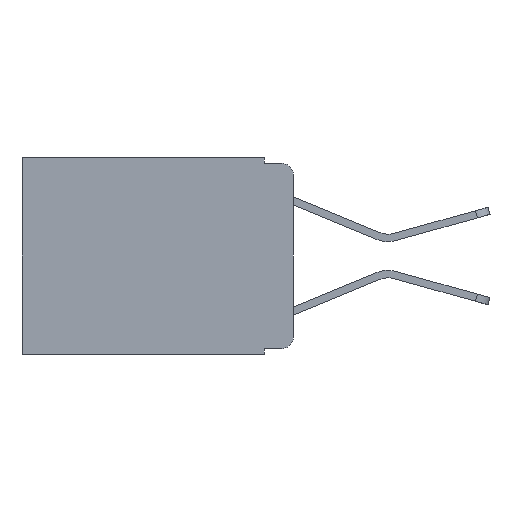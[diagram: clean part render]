
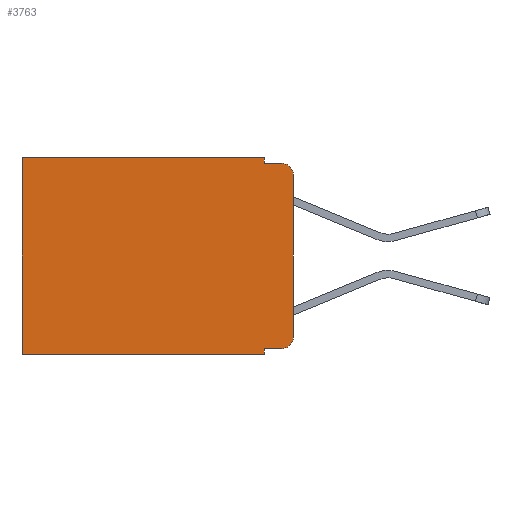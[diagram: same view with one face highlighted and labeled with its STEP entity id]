
A CAD part, left-side view. The second image highlights one B-rep face of the part: STEP entity #3763.
In plain terms, the highlighted planar face has unit normal (-1, 0, 0).
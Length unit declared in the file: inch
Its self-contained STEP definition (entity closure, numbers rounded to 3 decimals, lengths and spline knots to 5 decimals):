
#31 = ORIENTED_EDGE ( 'NONE', *, *, #11046, .F. ) ;
#92 = ORIENTED_EDGE ( 'NONE', *, *, #14139, .T. ) ;
#137 = CARTESIAN_POINT ( 'NONE',  ( 0.298, 0.051, -0.01 ) ) ;
#171 = ORIENTED_EDGE ( 'NONE', *, *, #2038, .T. ) ;
#335 = ORIENTED_EDGE ( 'NONE', *, *, #9919, .F. ) ;
#476 = VERTEX_POINT ( 'NONE', #11077 ) ;
#983 = LINE ( 'NONE', #5028, #12335 ) ;
#1116 = VECTOR ( 'NONE', #5757, 39.37008 ) ;
#1168 = EDGE_CURVE ( 'NONE', #7284, #14015, #10389, .T. ) ;
#1382 = DIRECTION ( 'NONE',  ( 0., 1., 0. ) ) ;
#1577 = DIRECTION ( 'NONE',  ( 0., 0., -1. ) ) ;
#1626 = VERTEX_POINT ( 'NONE', #10877 ) ;
#1864 = DIRECTION ( 'NONE',  ( 0., 1., 0. ) ) ;
#2035 = CARTESIAN_POINT ( 'NONE',  ( 0.298, 0.051, -0.333 ) ) ;
#2038 = EDGE_CURVE ( 'NONE', #14015, #6828, #9167, .T. ) ;
#2637 = CARTESIAN_POINT ( 'NONE',  ( 0.298, 0.473, 0. ) ) ;
#2832 = LINE ( 'NONE', #9396, #5446 ) ;
#3316 = CARTESIAN_POINT ( 'NONE',  ( 0.298, 0.051, -0.333 ) ) ;
#3537 = CARTESIAN_POINT ( 'NONE',  ( 0.298, 0.051, 0. ) ) ;
#3763 = ADVANCED_FACE ( 'NONE', ( #7193 ), #12557, .F. ) ;
#3995 = DIRECTION ( 'NONE',  ( 0., 0., -1. ) ) ;
#4475 = CARTESIAN_POINT ( 'NONE',  ( 0.298, 0., -0.313 ) ) ;
#4646 = ORIENTED_EDGE ( 'NONE', *, *, #6934, .T. ) ;
#4692 = CARTESIAN_POINT ( 'NONE',  ( 0.298, 0.02, -0.03 ) ) ;
#4764 = CARTESIAN_POINT ( 'NONE',  ( 0.298, 0.02, -0.333 ) ) ;
#4930 = VERTEX_POINT ( 'NONE', #6167 ) ;
#5028 = CARTESIAN_POINT ( 'NONE',  ( 0.298, 0., 0. ) ) ;
#5044 = CARTESIAN_POINT ( 'NONE',  ( 0.298, 0., -0.03 ) ) ;
#5356 = CARTESIAN_POINT ( 'NONE',  ( 0.298, 0., -0.343 ) ) ;
#5358 = DIRECTION ( 'NONE',  ( 0., -1., 0. ) ) ;
#5446 = VECTOR ( 'NONE', #1382, 39.37008 ) ;
#5665 = ORIENTED_EDGE ( 'NONE', *, *, #10648, .F. ) ;
#5757 = DIRECTION ( 'NONE',  ( 0., 0., -1. ) ) ;
#5793 = DIRECTION ( 'NONE',  ( 0., 0., -1. ) ) ;
#5821 = ORIENTED_EDGE ( 'NONE', *, *, #11369, .T. ) ;
#6073 = ORIENTED_EDGE ( 'NONE', *, *, #9181, .F. ) ;
#6122 = VECTOR ( 'NONE', #7340, 39.37008 ) ;
#6167 = CARTESIAN_POINT ( 'NONE',  ( 0.298, 0.051, 0. ) ) ;
#6828 = VERTEX_POINT ( 'NONE', #4475 ) ;
#6934 = EDGE_CURVE ( 'NONE', #13313, #1626, #14463, .T. ) ;
#7049 = CARTESIAN_POINT ( 'NONE',  ( 0.298, 0., 0. ) ) ;
#7151 = DIRECTION ( 'NONE',  ( 0., -1., 0. ) ) ;
#7193 = FACE_OUTER_BOUND ( 'NONE', #8470, .T. ) ;
#7284 = VERTEX_POINT ( 'NONE', #2035 ) ;
#7340 = DIRECTION ( 'NONE',  ( 0., 0., -1. ) ) ;
#7969 = VERTEX_POINT ( 'NONE', #137 ) ;
#8358 = LINE ( 'NONE', #5356, #14049 ) ;
#8434 = VERTEX_POINT ( 'NONE', #2637 ) ;
#8470 = EDGE_LOOP ( 'NONE', ( #6073, #4646, #335, #5665, #92, #5821, #31, #10484, #10145, #171 ) ) ;
#8568 = VECTOR ( 'NONE', #5358, 39.37008 ) ;
#9049 = VECTOR ( 'NONE', #1577, 39.37008 ) ;
#9135 = LINE ( 'NONE', #13785, #6122 ) ;
#9167 = CIRCLE ( 'NONE', #13107, 0.02 ) ;
#9181 = EDGE_CURVE ( 'NONE', #13313, #6828, #983, .T. ) ;
#9396 = CARTESIAN_POINT ( 'NONE',  ( 0.298, 0., 0. ) ) ;
#9565 = CARTESIAN_POINT ( 'NONE',  ( 0.298, 0.473, 0. ) ) ;
#9919 = EDGE_CURVE ( 'NONE', #7969, #1626, #11464, .T. ) ;
#9986 = VERTEX_POINT ( 'NONE', #11078 ) ;
#10145 = ORIENTED_EDGE ( 'NONE', *, *, #1168, .T. ) ;
#10262 = LINE ( 'NONE', #3537, #1116 ) ;
#10389 = LINE ( 'NONE', #3316, #12883 ) ;
#10484 = ORIENTED_EDGE ( 'NONE', *, *, #14188, .F. ) ;
#10648 = EDGE_CURVE ( 'NONE', #4930, #7969, #10262, .T. ) ;
#10877 = CARTESIAN_POINT ( 'NONE',  ( 0.298, 0.02, -0.01 ) ) ;
#11046 = EDGE_CURVE ( 'NONE', #476, #9986, #8358, .T. ) ;
#11077 = CARTESIAN_POINT ( 'NONE',  ( 0.298, 0.051, -0.343 ) ) ;
#11078 = CARTESIAN_POINT ( 'NONE',  ( 0.298, 0.473, -0.343 ) ) ;
#11369 = EDGE_CURVE ( 'NONE', #8434, #9986, #12270, .T. ) ;
#11464 = LINE ( 'NONE', #13046, #8568 ) ;
#11531 = AXIS2_PLACEMENT_3D ( 'NONE', #7049, #12390, #12439 ) ;
#12270 = LINE ( 'NONE', #9565, #9049 ) ;
#12335 = VECTOR ( 'NONE', #3995, 39.37008 ) ;
#12390 = DIRECTION ( 'NONE',  ( 1., 0., 0. ) ) ;
#12416 = DIRECTION ( 'NONE',  ( -1., 0., 0. ) ) ;
#12426 = CARTESIAN_POINT ( 'NONE',  ( 0.298, 0.02, -0.313 ) ) ;
#12439 = DIRECTION ( 'NONE',  ( 0., 0., -1. ) ) ;
#12455 = AXIS2_PLACEMENT_3D ( 'NONE', #4692, #12416, #5793 ) ;
#12557 = PLANE ( 'NONE',  #11531 ) ;
#12883 = VECTOR ( 'NONE', #7151, 39.37008 ) ;
#13046 = CARTESIAN_POINT ( 'NONE',  ( 0.298, 0.051, -0.01 ) ) ;
#13107 = AXIS2_PLACEMENT_3D ( 'NONE', #12426, #13922, #14008 ) ;
#13313 = VERTEX_POINT ( 'NONE', #5044 ) ;
#13785 = CARTESIAN_POINT ( 'NONE',  ( 0.298, 0.051, 0. ) ) ;
#13922 = DIRECTION ( 'NONE',  ( -1., 0., 0. ) ) ;
#14008 = DIRECTION ( 'NONE',  ( 0., 0., -1. ) ) ;
#14015 = VERTEX_POINT ( 'NONE', #4764 ) ;
#14049 = VECTOR ( 'NONE', #1864, 39.37008 ) ;
#14139 = EDGE_CURVE ( 'NONE', #4930, #8434, #2832, .T. ) ;
#14188 = EDGE_CURVE ( 'NONE', #7284, #476, #9135, .T. ) ;
#14463 = CIRCLE ( 'NONE', #12455, 0.02 ) ;
